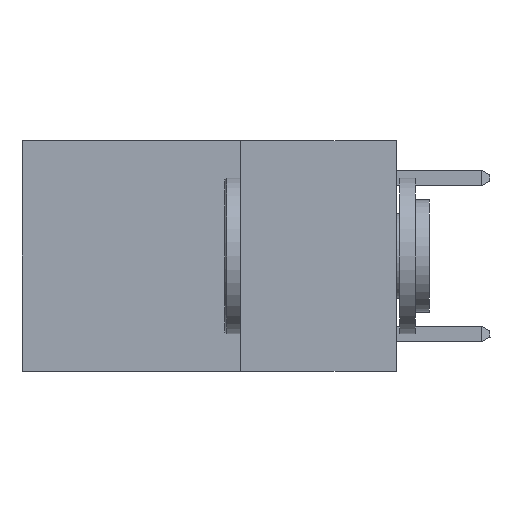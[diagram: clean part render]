
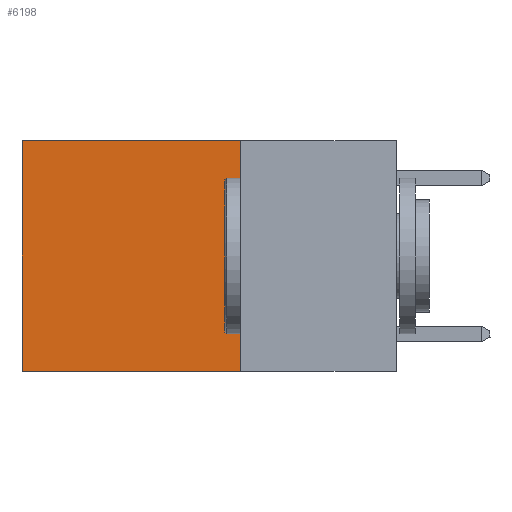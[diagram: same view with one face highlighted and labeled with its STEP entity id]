
A CAD part, left-side view. The second image highlights one B-rep face of the part: STEP entity #6198.
In plain terms, the highlighted planar face has unit normal (-1, 0, 0).
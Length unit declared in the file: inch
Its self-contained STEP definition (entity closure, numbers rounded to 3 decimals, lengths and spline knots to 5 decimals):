
#132 = VECTOR ( 'NONE', #3549, 39.37008 ) ;
#659 = CARTESIAN_POINT ( 'NONE',  ( 0.2625, 0.25, 0. ) ) ;
#1159 = VECTOR ( 'NONE', #1474, 39.37008 ) ;
#1185 = CARTESIAN_POINT ( 'NONE',  ( 0.2625, 0.25, 0. ) ) ;
#1377 = CARTESIAN_POINT ( 'NONE',  ( 0.2625, 0.6, 0. ) ) ;
#1474 = DIRECTION ( 'NONE',  ( 0., 0., -1. ) ) ;
#1603 = DIRECTION ( 'NONE',  ( 0., 1., 0. ) ) ;
#1816 = LINE ( 'NONE', #1377, #8759 ) ;
#2107 = DIRECTION ( 'NONE',  ( 0., 0., -1. ) ) ;
#2660 = CARTESIAN_POINT ( 'NONE',  ( 0.2625, 0.25, -0.37 ) ) ;
#2901 = CARTESIAN_POINT ( 'NONE',  ( 0.2625, 0.6, 0. ) ) ;
#3228 = FACE_OUTER_BOUND ( 'NONE', #4878, .T. ) ;
#3331 = LINE ( 'NONE', #6052, #1159 ) ;
#3339 = EDGE_CURVE ( 'NONE', #5680, #5622, #3331, .T. ) ;
#3549 = DIRECTION ( 'NONE',  ( 0., 1., 0. ) ) ;
#4878 = EDGE_LOOP ( 'NONE', ( #10664, #5779, #10249, #10316 ) ) ;
#4977 = EDGE_CURVE ( 'NONE', #6977, #6031, #1816, .T. ) ;
#5519 = CARTESIAN_POINT ( 'NONE',  ( 0.2625, 0.25, 0. ) ) ;
#5622 = VERTEX_POINT ( 'NONE', #2660 ) ;
#5680 = VERTEX_POINT ( 'NONE', #5519 ) ;
#5779 = ORIENTED_EDGE ( 'NONE', *, *, #6838, .F. ) ;
#5856 = AXIS2_PLACEMENT_3D ( 'NONE', #1185, #7655, #2107 ) ;
#6031 = VERTEX_POINT ( 'NONE', #8212 ) ;
#6052 = CARTESIAN_POINT ( 'NONE',  ( 0.2625, 0.25, 0. ) ) ;
#6198 = ADVANCED_FACE ( 'NONE', ( #3228 ), #9274, .F. ) ;
#6838 = EDGE_CURVE ( 'NONE', #5622, #6031, #7543, .T. ) ;
#6977 = VERTEX_POINT ( 'NONE', #2901 ) ;
#7447 = EDGE_CURVE ( 'NONE', #5680, #6977, #9849, .T. ) ;
#7543 = LINE ( 'NONE', #11221, #132 ) ;
#7655 = DIRECTION ( 'NONE',  ( 1., 0., 0. ) ) ;
#8212 = CARTESIAN_POINT ( 'NONE',  ( 0.2625, 0.6, -0.37 ) ) ;
#8221 = VECTOR ( 'NONE', #1603, 39.37008 ) ;
#8759 = VECTOR ( 'NONE', #10961, 39.37008 ) ;
#9274 = PLANE ( 'NONE',  #5856 ) ;
#9849 = LINE ( 'NONE', #659, #8221 ) ;
#10249 = ORIENTED_EDGE ( 'NONE', *, *, #3339, .F. ) ;
#10316 = ORIENTED_EDGE ( 'NONE', *, *, #7447, .T. ) ;
#10664 = ORIENTED_EDGE ( 'NONE', *, *, #4977, .T. ) ;
#10961 = DIRECTION ( 'NONE',  ( 0., 0., -1. ) ) ;
#11221 = CARTESIAN_POINT ( 'NONE',  ( 0.2625, 0.25, -0.37 ) ) ;
